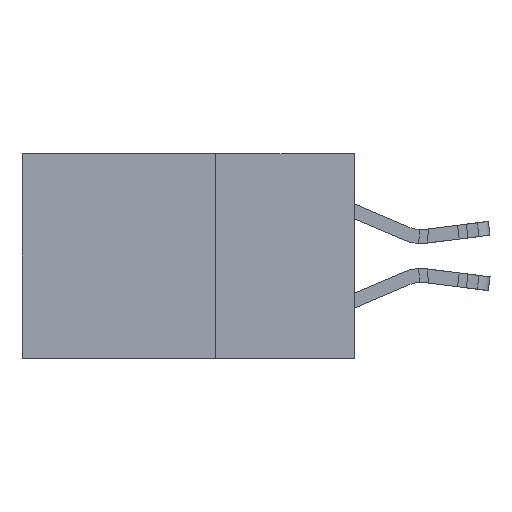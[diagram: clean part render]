
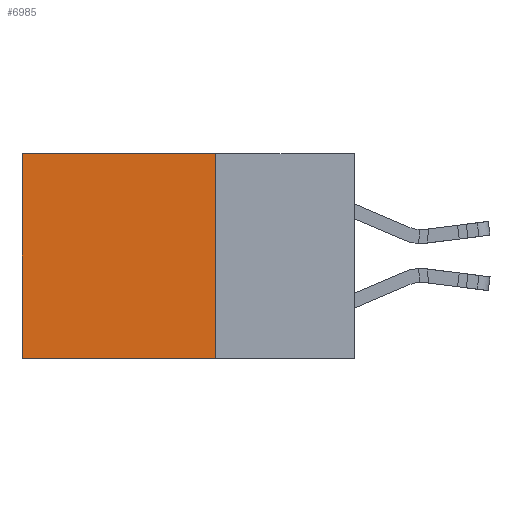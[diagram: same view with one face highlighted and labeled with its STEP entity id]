
A CAD part, left-side view. The second image highlights one B-rep face of the part: STEP entity #6985.
In plain terms, the highlighted planar face has unit normal (-1, 0, 0).
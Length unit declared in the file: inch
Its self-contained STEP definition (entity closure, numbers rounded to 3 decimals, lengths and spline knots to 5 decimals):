
#157 = EDGE_CURVE ( 'NONE', #7983, #5084, #7804, .T. ) ;
#923 = CARTESIAN_POINT ( 'NONE',  ( 0.298, 0.25, 0. ) ) ;
#968 = VERTEX_POINT ( 'NONE', #17510 ) ;
#1519 = EDGE_CURVE ( 'NONE', #968, #5084, #4351, .T. ) ;
#3074 = CARTESIAN_POINT ( 'NONE',  ( 0.298, 0.25, 0. ) ) ;
#3698 = VERTEX_POINT ( 'NONE', #923 ) ;
#4351 = LINE ( 'NONE', #27825, #23488 ) ;
#4401 = CARTESIAN_POINT ( 'NONE',  ( 0.298, 0.25, 0. ) ) ;
#5084 = VERTEX_POINT ( 'NONE', #14776 ) ;
#5971 = ORIENTED_EDGE ( 'NONE', *, *, #27015, .T. ) ;
#6045 = CARTESIAN_POINT ( 'NONE',  ( 0.298, 0.6, 0. ) ) ;
#6985 = ADVANCED_FACE ( 'NONE', ( #15674 ), #8214, .F. ) ;
#7804 = LINE ( 'NONE', #6045, #19003 ) ;
#7983 = VERTEX_POINT ( 'NONE', #24127 ) ;
#8214 = PLANE ( 'NONE',  #20839 ) ;
#13395 = CARTESIAN_POINT ( 'NONE',  ( 0.298, 0.25, 0. ) ) ;
#14776 = CARTESIAN_POINT ( 'NONE',  ( 0.298, 0.6, -0.37 ) ) ;
#15498 = ORIENTED_EDGE ( 'NONE', *, *, #157, .T. ) ;
#15674 = FACE_OUTER_BOUND ( 'NONE', #25350, .T. ) ;
#15854 = DIRECTION ( 'NONE',  ( 0., 0., -1. ) ) ;
#16629 = LINE ( 'NONE', #13395, #29388 ) ;
#17510 = CARTESIAN_POINT ( 'NONE',  ( 0.298, 0.25, -0.37 ) ) ;
#17702 = EDGE_CURVE ( 'NONE', #3698, #968, #16629, .T. ) ;
#17831 = DIRECTION ( 'NONE',  ( 1., 0., 0. ) ) ;
#19003 = VECTOR ( 'NONE', #15854, 39.37008 ) ;
#19838 = DIRECTION ( 'NONE',  ( 0., 0., -1. ) ) ;
#20288 = LINE ( 'NONE', #4401, #25882 ) ;
#20645 = DIRECTION ( 'NONE',  ( 0., 0., -1. ) ) ;
#20723 = DIRECTION ( 'NONE',  ( 0., 1., 0. ) ) ;
#20839 = AXIS2_PLACEMENT_3D ( 'NONE', #3074, #17831, #19838 ) ;
#23488 = VECTOR ( 'NONE', #20723, 39.37008 ) ;
#24127 = CARTESIAN_POINT ( 'NONE',  ( 0.298, 0.6, 0. ) ) ;
#24623 = ORIENTED_EDGE ( 'NONE', *, *, #17702, .F. ) ;
#25350 = EDGE_LOOP ( 'NONE', ( #15498, #29118, #24623, #5971 ) ) ;
#25882 = VECTOR ( 'NONE', #26009, 39.37008 ) ;
#26009 = DIRECTION ( 'NONE',  ( 0., 1., 0. ) ) ;
#27015 = EDGE_CURVE ( 'NONE', #3698, #7983, #20288, .T. ) ;
#27825 = CARTESIAN_POINT ( 'NONE',  ( 0.298, 0.25, -0.37 ) ) ;
#29118 = ORIENTED_EDGE ( 'NONE', *, *, #1519, .F. ) ;
#29388 = VECTOR ( 'NONE', #20645, 39.37008 ) ;
